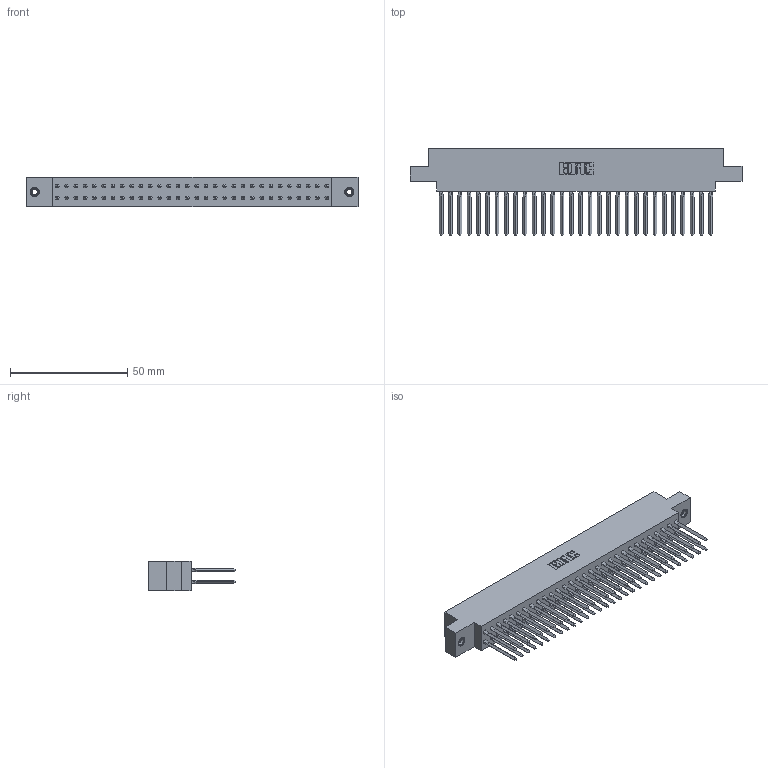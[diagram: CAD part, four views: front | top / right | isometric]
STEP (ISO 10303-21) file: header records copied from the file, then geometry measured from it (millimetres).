
FILE_DESCRIPTION (( 'STEP AP203' ), '1' );
FILE_NAME ('317-060-542-878.STEP', '2020-02-28T05:10:01', ( '' ), ( '' ), 'SwSTEP 2.0', 'SolidWorks 2016', '' );
FILE_SCHEMA (( 'CONFIG_CONTROL_DESIGN' ));
Length unit declared in the file: inch
Products named in the file (4): 317 Part_.156 Dia - TI; 345-250-001_345-250-003-102; 317-060-542-878; 317-290-003_542
Assembly tree (63 placements, depth 2):
  317-060-542-878
    317 Part_.156 Dia - TI
    317-290-003_542  x60
    345-250-001_345-250-003-102  x2
Bounding box: 141.58 x 37.34 x 12.7 mm (x, y, z)
Volume: 22797.4 mm3; surface area: 31339.4 mm2
Topology: 63 solids, 63 shells, 3582 faces, 10011 edges, 6386 vertices
Faces by surface type: plane 2850, cylinder 476, bspline 240, cone 12, torus 4
Entity records: 45242 total; most frequent: CARTESIAN_POINT 8112, ORIENTED_EDGE 7768, DIRECTION 6594, EDGE_CURVE 3884, VECTOR 3694, LINE 3694, VERTEX_POINT 2580, AXIS2_PLACEMENT_3D 1450
